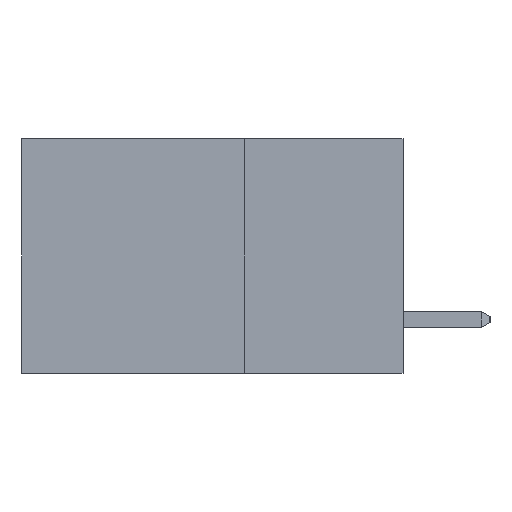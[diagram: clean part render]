
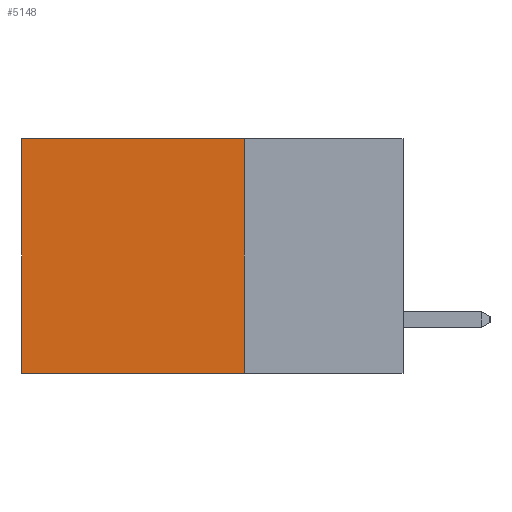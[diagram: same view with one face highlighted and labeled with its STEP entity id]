
A CAD part, left-side view. The second image highlights one B-rep face of the part: STEP entity #5148.
In plain terms, the highlighted planar face has unit normal (-1, 0, 0).
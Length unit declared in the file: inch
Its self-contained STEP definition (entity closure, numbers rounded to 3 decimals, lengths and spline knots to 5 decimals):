
#456 = VECTOR ( 'NONE', #16068, 39.37008 ) ;
#1320 = EDGE_CURVE ( 'NONE', #19304, #8101, #8415, .T. ) ;
#1593 = VECTOR ( 'NONE', #8544, 39.37008 ) ;
#3130 = LINE ( 'NONE', #18977, #20368 ) ;
#3285 = CARTESIAN_POINT ( 'NONE',  ( 0.2875, 0.25, 0. ) ) ;
#4416 = LINE ( 'NONE', #9350, #456 ) ;
#4694 = CARTESIAN_POINT ( 'NONE',  ( 0.2875, 0.6, 0. ) ) ;
#4927 = ORIENTED_EDGE ( 'NONE', *, *, #1320, .T. ) ;
#5148 = ADVANCED_FACE ( 'NONE', ( #5283 ), #13456, .F. ) ;
#5226 = CARTESIAN_POINT ( 'NONE',  ( 0.2875, 0.6, -0.37 ) ) ;
#5283 = FACE_OUTER_BOUND ( 'NONE', #5580, .T. ) ;
#5297 = CARTESIAN_POINT ( 'NONE',  ( 0.2875, 0.25, 0. ) ) ;
#5497 = ORIENTED_EDGE ( 'NONE', *, *, #6624, .F. ) ;
#5580 = EDGE_LOOP ( 'NONE', ( #4927, #5497, #7584, #21603 ) ) ;
#6624 = EDGE_CURVE ( 'NONE', #12945, #8101, #3130, .T. ) ;
#6717 = DIRECTION ( 'NONE',  ( 0., 0., -1. ) ) ;
#7081 = CARTESIAN_POINT ( 'NONE',  ( 0.2875, 0.6, 0. ) ) ;
#7584 = ORIENTED_EDGE ( 'NONE', *, *, #8491, .F. ) ;
#8101 = VERTEX_POINT ( 'NONE', #5226 ) ;
#8408 = DIRECTION ( 'NONE',  ( 1., 0., 0. ) ) ;
#8415 = LINE ( 'NONE', #7081, #1593 ) ;
#8491 = EDGE_CURVE ( 'NONE', #20430, #12945, #4416, .T. ) ;
#8544 = DIRECTION ( 'NONE',  ( 0., 0., -1. ) ) ;
#8634 = CARTESIAN_POINT ( 'NONE',  ( 0.2875, 0.25, 0. ) ) ;
#9350 = CARTESIAN_POINT ( 'NONE',  ( 0.2875, 0.25, 0. ) ) ;
#9654 = DIRECTION ( 'NONE',  ( 0., 1., 0. ) ) ;
#11416 = AXIS2_PLACEMENT_3D ( 'NONE', #8634, #8408, #6717 ) ;
#12290 = CARTESIAN_POINT ( 'NONE',  ( 0.2875, 0.25, -0.37 ) ) ;
#12945 = VERTEX_POINT ( 'NONE', #12290 ) ;
#13456 = PLANE ( 'NONE',  #11416 ) ;
#15776 = DIRECTION ( 'NONE',  ( 0., 1., 0. ) ) ;
#16068 = DIRECTION ( 'NONE',  ( 0., 0., -1. ) ) ;
#17718 = VECTOR ( 'NONE', #9654, 39.37008 ) ;
#18977 = CARTESIAN_POINT ( 'NONE',  ( 0.2875, 0.25, -0.37 ) ) ;
#19040 = LINE ( 'NONE', #5297, #17718 ) ;
#19304 = VERTEX_POINT ( 'NONE', #4694 ) ;
#19815 = EDGE_CURVE ( 'NONE', #20430, #19304, #19040, .T. ) ;
#20368 = VECTOR ( 'NONE', #15776, 39.37008 ) ;
#20430 = VERTEX_POINT ( 'NONE', #3285 ) ;
#21603 = ORIENTED_EDGE ( 'NONE', *, *, #19815, .T. ) ;
